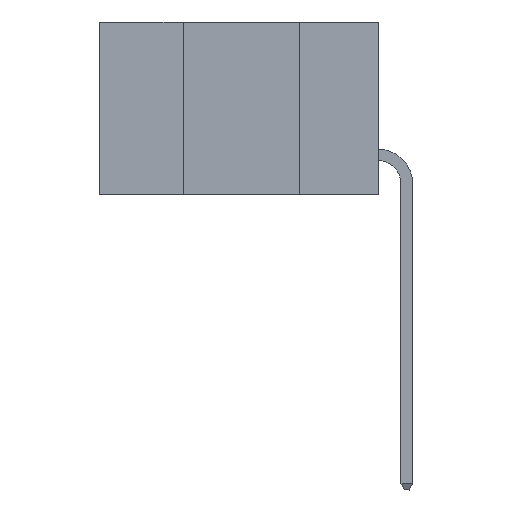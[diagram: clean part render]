
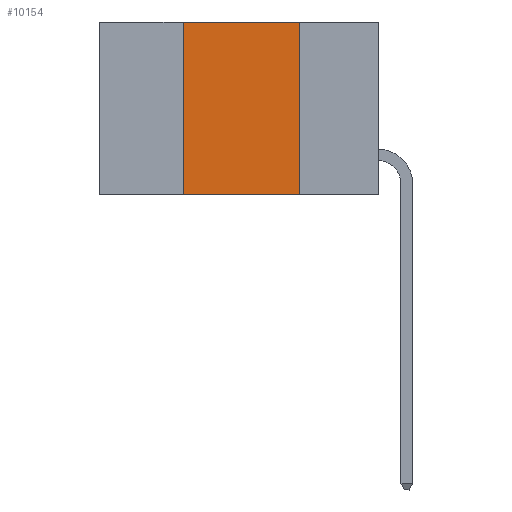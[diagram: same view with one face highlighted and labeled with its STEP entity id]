
A CAD part, left-side view. The second image highlights one B-rep face of the part: STEP entity #10154.
In plain terms, the highlighted planar face has unit normal (-1, 0, 0).
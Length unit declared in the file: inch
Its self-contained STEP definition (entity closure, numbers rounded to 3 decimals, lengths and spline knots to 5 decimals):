
#105 = VERTEX_POINT ( 'NONE', #8930 ) ;
#267 = EDGE_CURVE ( 'NONE', #3230, #4019, #10028, .T. ) ;
#374 = FACE_OUTER_BOUND ( 'NONE', #7323, .T. ) ;
#2128 = ORIENTED_EDGE ( 'NONE', *, *, #267, .F. ) ;
#2359 = CARTESIAN_POINT ( 'NONE',  ( 0., 0.6, -0.37 ) ) ;
#2754 = DIRECTION ( 'NONE',  ( 1., 0., 0. ) ) ;
#2999 = VECTOR ( 'NONE', #9290, 39.37008 ) ;
#3151 = AXIS2_PLACEMENT_3D ( 'NONE', #6725, #2754, #5932 ) ;
#3230 = VERTEX_POINT ( 'NONE', #8850 ) ;
#3231 = ORIENTED_EDGE ( 'NONE', *, *, #8023, .F. ) ;
#3480 = PLANE ( 'NONE',  #3151 ) ;
#3669 = DIRECTION ( 'NONE',  ( 0., 0., 1. ) ) ;
#3816 = CARTESIAN_POINT ( 'NONE',  ( 0., 0.6, 0. ) ) ;
#4019 = VERTEX_POINT ( 'NONE', #9047 ) ;
#4056 = DIRECTION ( 'NONE',  ( 0., -1., 0. ) ) ;
#4553 = CARTESIAN_POINT ( 'NONE',  ( 0., 0.17, -0.37 ) ) ;
#4618 = VECTOR ( 'NONE', #4056, 39.37008 ) ;
#5167 = VECTOR ( 'NONE', #3669, 39.37008 ) ;
#5932 = DIRECTION ( 'NONE',  ( 0., 0., -1. ) ) ;
#6415 = VERTEX_POINT ( 'NONE', #7223 ) ;
#6725 = CARTESIAN_POINT ( 'NONE',  ( 0., 0.6, 0. ) ) ;
#6908 = EDGE_CURVE ( 'NONE', #6415, #4019, #9460, .T. ) ;
#6960 = DIRECTION ( 'NONE',  ( 0., -1., 0. ) ) ;
#6969 = VECTOR ( 'NONE', #6960, 39.37008 ) ;
#7201 = ORIENTED_EDGE ( 'NONE', *, *, #9418, .F. ) ;
#7223 = CARTESIAN_POINT ( 'NONE',  ( 0., 0.42, -0.37 ) ) ;
#7323 = EDGE_LOOP ( 'NONE', ( #2128, #3231, #7201, #10119 ) ) ;
#7529 = LINE ( 'NONE', #9880, #5167 ) ;
#8023 = EDGE_CURVE ( 'NONE', #105, #3230, #9353, .T. ) ;
#8850 = CARTESIAN_POINT ( 'NONE',  ( 0., 0.17, 0. ) ) ;
#8930 = CARTESIAN_POINT ( 'NONE',  ( 0., 0.42, 0. ) ) ;
#9047 = CARTESIAN_POINT ( 'NONE',  ( 0., 0.17, -0.37 ) ) ;
#9290 = DIRECTION ( 'NONE',  ( 0., 0., -1. ) ) ;
#9353 = LINE ( 'NONE', #3816, #6969 ) ;
#9418 = EDGE_CURVE ( 'NONE', #6415, #105, #7529, .T. ) ;
#9460 = LINE ( 'NONE', #2359, #4618 ) ;
#9880 = CARTESIAN_POINT ( 'NONE',  ( 0., 0.42, -0.37 ) ) ;
#10028 = LINE ( 'NONE', #4553, #2999 ) ;
#10119 = ORIENTED_EDGE ( 'NONE', *, *, #6908, .T. ) ;
#10154 = ADVANCED_FACE ( 'NONE', ( #374 ), #3480, .F. ) ;
